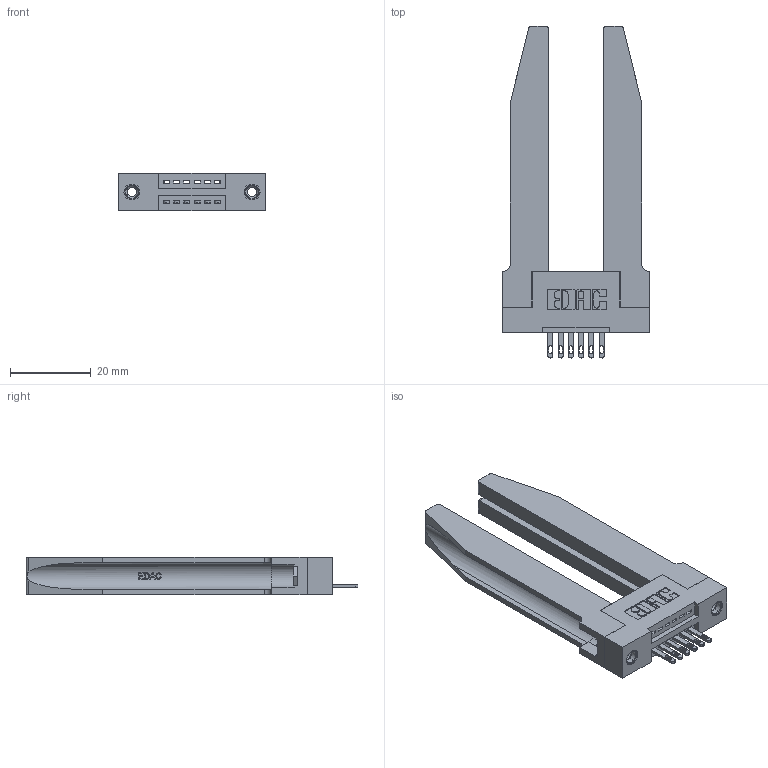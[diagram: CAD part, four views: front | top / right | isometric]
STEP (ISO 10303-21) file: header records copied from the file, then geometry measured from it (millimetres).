
FILE_DESCRIPTION (( 'STEP AP203' ), '1' );
FILE_NAME ('345-006-500-178.STEP', '2019-10-03T15:01:07', ( '' ), ( '' ), 'SwSTEP 2.0', 'SolidWorks 2016', '' );
FILE_SCHEMA (( 'CONFIG_CONTROL_DESIGN' ));
Length unit declared in the file: inch
Products named in the file (5): 345-220-078_345-220-078; 345-292-001_345-293-100; 345-006-500-178; 345-250-001_345-250-001-102; 345 Part_Flush Mounting Lugs - 0.156 Dia-TH
Assembly tree (11 placements, depth 2):
  345-006-500-178
    345 Part_Flush Mounting Lugs - 0.156 Dia-TH
    345-292-001_345-293-100  x6
    345-250-001_345-250-001-102  x2
    345-220-078_345-220-078  x2
Bounding box: 36.47 x 82.47 x 9.4 mm (x, y, z)
Volume: 10943.7 mm3; surface area: 10586.7 mm2
Topology: 11 solids, 11 shells, 684 faces, 1957 edges, 1294 vertices
Faces by surface type: plane 426, cylinder 206, bspline 36, cone 12, torus 4
Entity records: 14032 total; most frequent: CARTESIAN_POINT 3329, ORIENTED_EDGE 2166, DIRECTION 1969, EDGE_CURVE 1083, VECTOR 829, LINE 829, VERTEX_POINT 716, AXIS2_PLACEMENT_3D 570
